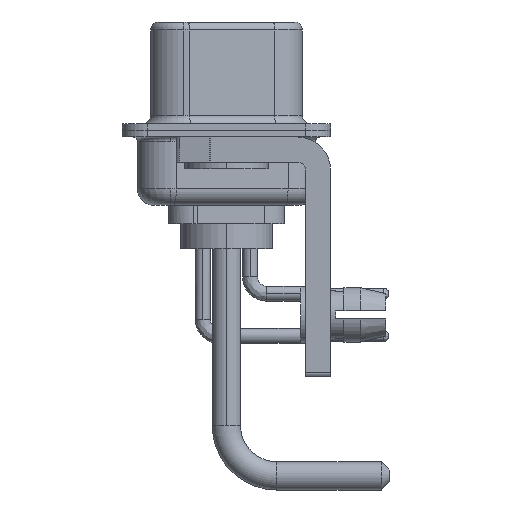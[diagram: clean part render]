
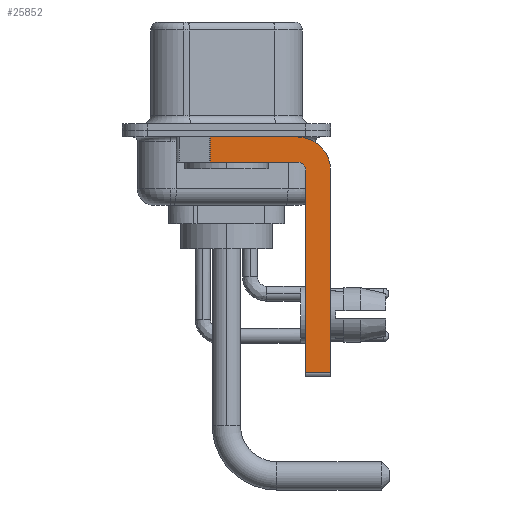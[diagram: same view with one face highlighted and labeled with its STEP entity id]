
A CAD part, left-side view. The second image highlights one B-rep face of the part: STEP entity #25852.
In plain terms, the highlighted planar face has unit normal (-1, 0, 0).
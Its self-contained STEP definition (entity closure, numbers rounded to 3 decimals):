
#406 = DIRECTION ( 'NONE',  ( 0., -1., 0. ) ) ;
#667 = LINE ( 'NONE', #13581, #26748 ) ;
#1012 = ORIENTED_EDGE ( 'NONE', *, *, #20132, .F. ) ;
#1477 = DIRECTION ( 'NONE',  ( 1., 0., 0. ) ) ;
#1528 = ORIENTED_EDGE ( 'NONE', *, *, #13404, .F. ) ;
#1961 = EDGE_LOOP ( 'NONE', ( #15153, #24571, #1012, #26208, #19160, #9687, #1528, #15532 ) ) ;
#2775 = CIRCLE ( 'NONE', #12717, 0.5 ) ;
#3856 = VERTEX_POINT ( 'NONE', #12335 ) ;
#4165 = VERTEX_POINT ( 'NONE', #26757 ) ;
#4325 = CARTESIAN_POINT ( 'NONE',  ( -2.9, -4.25, -2.4 ) ) ;
#4784 = AXIS2_PLACEMENT_3D ( 'NONE', #16354, #24974, #14226 ) ;
#5586 = CARTESIAN_POINT ( 'NONE',  ( -2.9, -4.75, -14.55 ) ) ;
#5811 = VECTOR ( 'NONE', #8697, 1000. ) ;
#6262 = VECTOR ( 'NONE', #406, 1000. ) ;
#6721 = CARTESIAN_POINT ( 'NONE',  ( -2.9, -6.25, -14.55 ) ) ;
#6842 = VERTEX_POINT ( 'NONE', #9357 ) ;
#7014 = VECTOR ( 'NONE', #17213, 1000. ) ;
#8055 = CARTESIAN_POINT ( 'NONE',  ( -2.9, -4.25, -1.9 ) ) ;
#8588 = LINE ( 'NONE', #12542, #7014 ) ;
#8677 = CARTESIAN_POINT ( 'NONE',  ( -2.9, -4.25, -1.9 ) ) ;
#8697 = DIRECTION ( 'NONE',  ( 0., 0., -1. ) ) ;
#8710 = EDGE_CURVE ( 'NONE', #8979, #26479, #2775, .T. ) ;
#8837 = VERTEX_POINT ( 'NONE', #6721 ) ;
#8979 = VERTEX_POINT ( 'NONE', #27233 ) ;
#9209 = LINE ( 'NONE', #19815, #6262 ) ;
#9357 = CARTESIAN_POINT ( 'NONE',  ( -2.9, -6.25, -2.4 ) ) ;
#9687 = ORIENTED_EDGE ( 'NONE', *, *, #14961, .T. ) ;
#10960 = CARTESIAN_POINT ( 'NONE',  ( -2.9, 0.978, -1.9 ) ) ;
#12335 = CARTESIAN_POINT ( 'NONE',  ( -2.9, 0.978, -1.9 ) ) ;
#12394 = VERTEX_POINT ( 'NONE', #14057 ) ;
#12479 = CIRCLE ( 'NONE', #4784, 2. ) ;
#12542 = CARTESIAN_POINT ( 'NONE',  ( -2.9, -4.25, -14.55 ) ) ;
#12717 = AXIS2_PLACEMENT_3D ( 'NONE', #4325, #16649, #21027 ) ;
#13404 = EDGE_CURVE ( 'NONE', #6842, #8837, #18641, .T. ) ;
#13581 = CARTESIAN_POINT ( 'NONE',  ( -2.9, -4.75, -14.8 ) ) ;
#13885 = VECTOR ( 'NONE', #22607, 1000. ) ;
#14057 = CARTESIAN_POINT ( 'NONE',  ( -2.9, 0.978, -0.4 ) ) ;
#14165 = LINE ( 'NONE', #8055, #23927 ) ;
#14226 = DIRECTION ( 'NONE',  ( 0., 0., -1. ) ) ;
#14254 = CARTESIAN_POINT ( 'NONE',  ( -2.9, -6.25, -2.4 ) ) ;
#14961 = EDGE_CURVE ( 'NONE', #22738, #8837, #8588, .T. ) ;
#15153 = ORIENTED_EDGE ( 'NONE', *, *, #19927, .F. ) ;
#15290 = EDGE_CURVE ( 'NONE', #4165, #6842, #12479, .T. ) ;
#15532 = ORIENTED_EDGE ( 'NONE', *, *, #15290, .F. ) ;
#16354 = CARTESIAN_POINT ( 'NONE',  ( -2.9, -4.25, -2.4 ) ) ;
#16500 = CARTESIAN_POINT ( 'NONE',  ( -2.9, -4.25, -2.4 ) ) ;
#16639 = DIRECTION ( 'NONE',  ( 0., 0., -1. ) ) ;
#16649 = DIRECTION ( 'NONE',  ( -1., 0., 0. ) ) ;
#17213 = DIRECTION ( 'NONE',  ( 0., -1., 0. ) ) ;
#18641 = LINE ( 'NONE', #14254, #13885 ) ;
#19160 = ORIENTED_EDGE ( 'NONE', *, *, #23947, .F. ) ;
#19815 = CARTESIAN_POINT ( 'NONE',  ( -2.9, 3., -0.4 ) ) ;
#19927 = EDGE_CURVE ( 'NONE', #12394, #4165, #9209, .T. ) ;
#20132 = EDGE_CURVE ( 'NONE', #26479, #3856, #14165, .T. ) ;
#20183 = PLANE ( 'NONE',  #24275 ) ;
#21027 = DIRECTION ( 'NONE',  ( 0., 0., 1. ) ) ;
#22607 = DIRECTION ( 'NONE',  ( 0., 0., -1. ) ) ;
#22738 = VERTEX_POINT ( 'NONE', #5586 ) ;
#23187 = DIRECTION ( 'NONE',  ( 0., 1., 0. ) ) ;
#23548 = LINE ( 'NONE', #10960, #5811 ) ;
#23927 = VECTOR ( 'NONE', #23187, 1000. ) ;
#23947 = EDGE_CURVE ( 'NONE', #22738, #8979, #667, .T. ) ;
#24275 = AXIS2_PLACEMENT_3D ( 'NONE', #16500, #1477, #16639 ) ;
#24571 = ORIENTED_EDGE ( 'NONE', *, *, #27382, .T. ) ;
#24974 = DIRECTION ( 'NONE',  ( 1., 0., 0. ) ) ;
#25852 = ADVANCED_FACE ( 'NONE', ( #26422 ), #20183, .F. ) ;
#26208 = ORIENTED_EDGE ( 'NONE', *, *, #8710, .F. ) ;
#26422 = FACE_OUTER_BOUND ( 'NONE', #1961, .T. ) ;
#26479 = VERTEX_POINT ( 'NONE', #8677 ) ;
#26748 = VECTOR ( 'NONE', #27010, 1000. ) ;
#26757 = CARTESIAN_POINT ( 'NONE',  ( -2.9, -4.25, -0.4 ) ) ;
#27010 = DIRECTION ( 'NONE',  ( 0., 0., 1. ) ) ;
#27233 = CARTESIAN_POINT ( 'NONE',  ( -2.9, -4.75, -2.4 ) ) ;
#27382 = EDGE_CURVE ( 'NONE', #12394, #3856, #23548, .T. ) ;
